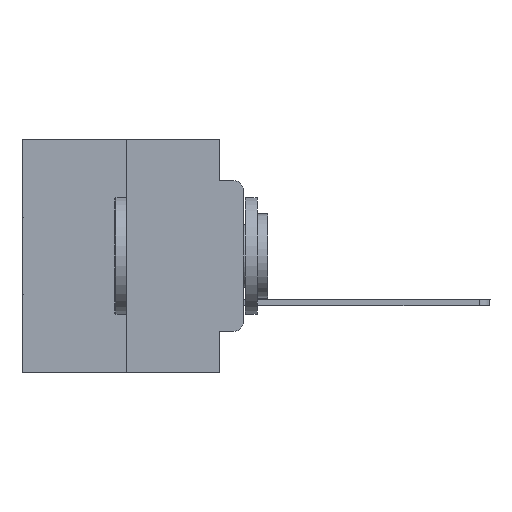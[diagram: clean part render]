
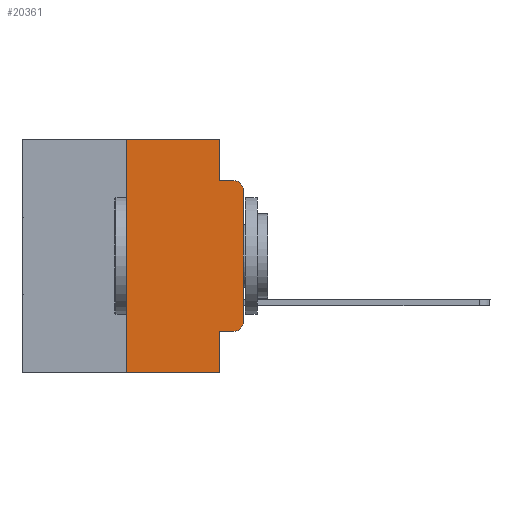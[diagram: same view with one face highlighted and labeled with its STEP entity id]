
A CAD part, left-side view. The second image highlights one B-rep face of the part: STEP entity #20361.
In plain terms, the highlighted planar face has unit normal (-1, 0, 0).
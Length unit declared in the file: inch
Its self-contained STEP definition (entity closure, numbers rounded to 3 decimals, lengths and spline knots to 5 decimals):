
#843 = VERTEX_POINT ( 'NONE', #23609 ) ;
#894 = VERTEX_POINT ( 'NONE', #10876 ) ;
#933 = LINE ( 'NONE', #22660, #13069 ) ;
#1000 = ORIENTED_EDGE ( 'NONE', *, *, #3573, .F. ) ;
#1607 = DIRECTION ( 'NONE',  ( -1., 0., 0. ) ) ;
#2067 = DIRECTION ( 'NONE',  ( 0., 0., -1. ) ) ;
#2489 = VERTEX_POINT ( 'NONE', #3568 ) ;
#2882 = LINE ( 'NONE', #15921, #21929 ) ;
#3162 = EDGE_CURVE ( 'NONE', #894, #11523, #4607, .T. ) ;
#3229 = VECTOR ( 'NONE', #24380, 39.37008 ) ;
#3568 = CARTESIAN_POINT ( 'NONE',  ( 0., 0., -0.1085 ) ) ;
#3573 = EDGE_CURVE ( 'NONE', #27974, #17882, #2882, .T. ) ;
#3927 = CARTESIAN_POINT ( 'NONE',  ( 0., 0.473, -0.5 ) ) ;
#4607 = CIRCLE ( 'NONE', #15138, 0.02 ) ;
#5653 = VECTOR ( 'NONE', #20807, 39.37008 ) ;
#5992 = VECTOR ( 'NONE', #17381, 39.37008 ) ;
#7001 = CARTESIAN_POINT ( 'NONE',  ( 0., 0.02, -0.0885 ) ) ;
#7989 = CARTESIAN_POINT ( 'NONE',  ( 0., 0.051, 0. ) ) ;
#8344 = LINE ( 'NONE', #3927, #26092 ) ;
#8503 = DIRECTION ( 'NONE',  ( 1., 0., 0. ) ) ;
#8658 = LINE ( 'NONE', #25150, #5992 ) ;
#9084 = LINE ( 'NONE', #26520, #3229 ) ;
#9503 = CARTESIAN_POINT ( 'NONE',  ( 0., 0.051, -0.5 ) ) ;
#9590 = EDGE_CURVE ( 'NONE', #24425, #843, #9084, .T. ) ;
#9621 = VERTEX_POINT ( 'NONE', #9503 ) ;
#10326 = DIRECTION ( 'NONE',  ( 0., 0., -1. ) ) ;
#10332 = EDGE_CURVE ( 'NONE', #2489, #17882, #25646, .T. ) ;
#10384 = ORIENTED_EDGE ( 'NONE', *, *, #24829, .F. ) ;
#10876 = CARTESIAN_POINT ( 'NONE',  ( 0., 0.02, -0.4115 ) ) ;
#11523 = VERTEX_POINT ( 'NONE', #13654 ) ;
#11677 = VERTEX_POINT ( 'NONE', #21887 ) ;
#11712 = ORIENTED_EDGE ( 'NONE', *, *, #25781, .F. ) ;
#11790 = CARTESIAN_POINT ( 'NONE',  ( 0., 0.02, -0.3915 ) ) ;
#11811 = DIRECTION ( 'NONE',  ( 0., -1., 0. ) ) ;
#11974 = EDGE_LOOP ( 'NONE', ( #19119, #15191, #1000, #10384, #18674, #20425, #21618, #11712, #13873, #15837 ) ) ;
#12474 = CARTESIAN_POINT ( 'NONE',  ( 0., 0.02, -0.1085 ) ) ;
#13069 = VECTOR ( 'NONE', #11811, 39.37008 ) ;
#13654 = CARTESIAN_POINT ( 'NONE',  ( 0., 0., -0.3915 ) ) ;
#13873 = ORIENTED_EDGE ( 'NONE', *, *, #20885, .T. ) ;
#14187 = AXIS2_PLACEMENT_3D ( 'NONE', #23942, #8503, #23802 ) ;
#14236 = DIRECTION ( 'NONE',  ( 0., 0., 1. ) ) ;
#14246 = VERTEX_POINT ( 'NONE', #7989 ) ;
#15138 = AXIS2_PLACEMENT_3D ( 'NONE', #11790, #20359, #19944 ) ;
#15191 = ORIENTED_EDGE ( 'NONE', *, *, #10332, .T. ) ;
#15556 = VECTOR ( 'NONE', #14236, 39.37008 ) ;
#15837 = ORIENTED_EDGE ( 'NONE', *, *, #3162, .T. ) ;
#15921 = CARTESIAN_POINT ( 'NONE',  ( 0., 0.051, -0.0885 ) ) ;
#16099 = LINE ( 'NONE', #17951, #15556 ) ;
#16533 = LINE ( 'NONE', #18947, #5653 ) ;
#16791 = DIRECTION ( 'NONE',  ( 0., -1., 0. ) ) ;
#17381 = DIRECTION ( 'NONE',  ( 0., -1., 0. ) ) ;
#17882 = VERTEX_POINT ( 'NONE', #7001 ) ;
#17951 = CARTESIAN_POINT ( 'NONE',  ( 0., 0., 0. ) ) ;
#18674 = ORIENTED_EDGE ( 'NONE', *, *, #26838, .F. ) ;
#18947 = CARTESIAN_POINT ( 'NONE',  ( 0., 0.051, 0. ) ) ;
#19119 = ORIENTED_EDGE ( 'NONE', *, *, #20033, .T. ) ;
#19944 = DIRECTION ( 'NONE',  ( 0., 0., -1. ) ) ;
#20033 = EDGE_CURVE ( 'NONE', #11523, #2489, #16099, .T. ) ;
#20359 = DIRECTION ( 'NONE',  ( -1., 0., 0. ) ) ;
#20361 = ADVANCED_FACE ( 'NONE', ( #22060 ), #26362, .F. ) ;
#20425 = ORIENTED_EDGE ( 'NONE', *, *, #9590, .F. ) ;
#20794 = LINE ( 'NONE', #21651, #22563 ) ;
#20807 = DIRECTION ( 'NONE',  ( 0., 0., -1. ) ) ;
#20885 = EDGE_CURVE ( 'NONE', #11677, #894, #8658, .T. ) ;
#21166 = CARTESIAN_POINT ( 'NONE',  ( 0., 0.051, -0.0885 ) ) ;
#21388 = EDGE_CURVE ( 'NONE', #24425, #9621, #8344, .T. ) ;
#21618 = ORIENTED_EDGE ( 'NONE', *, *, #21388, .T. ) ;
#21651 = CARTESIAN_POINT ( 'NONE',  ( 0., 0.051, 0. ) ) ;
#21887 = CARTESIAN_POINT ( 'NONE',  ( 0., 0.051, -0.4115 ) ) ;
#21929 = VECTOR ( 'NONE', #26758, 39.37008 ) ;
#22060 = FACE_OUTER_BOUND ( 'NONE', #11974, .T. ) ;
#22563 = VECTOR ( 'NONE', #2067, 39.37008 ) ;
#22660 = CARTESIAN_POINT ( 'NONE',  ( 0., 0.473, 0. ) ) ;
#23609 = CARTESIAN_POINT ( 'NONE',  ( 0., 0.25, 0. ) ) ;
#23802 = DIRECTION ( 'NONE',  ( 0., 0., -1. ) ) ;
#23815 = AXIS2_PLACEMENT_3D ( 'NONE', #12474, #1607, #10326 ) ;
#23942 = CARTESIAN_POINT ( 'NONE',  ( 0., 0.473, 0. ) ) ;
#24380 = DIRECTION ( 'NONE',  ( 0., 0., 1. ) ) ;
#24425 = VERTEX_POINT ( 'NONE', #25755 ) ;
#24829 = EDGE_CURVE ( 'NONE', #14246, #27974, #16533, .T. ) ;
#25150 = CARTESIAN_POINT ( 'NONE',  ( 0., 0.051, -0.4115 ) ) ;
#25646 = CIRCLE ( 'NONE', #23815, 0.02 ) ;
#25755 = CARTESIAN_POINT ( 'NONE',  ( 0., 0.25, -0.5 ) ) ;
#25781 = EDGE_CURVE ( 'NONE', #11677, #9621, #20794, .T. ) ;
#26092 = VECTOR ( 'NONE', #16791, 39.37008 ) ;
#26362 = PLANE ( 'NONE',  #14187 ) ;
#26520 = CARTESIAN_POINT ( 'NONE',  ( 0., 0.25, 0. ) ) ;
#26758 = DIRECTION ( 'NONE',  ( 0., -1., 0. ) ) ;
#26838 = EDGE_CURVE ( 'NONE', #843, #14246, #933, .T. ) ;
#27974 = VERTEX_POINT ( 'NONE', #21166 ) ;
